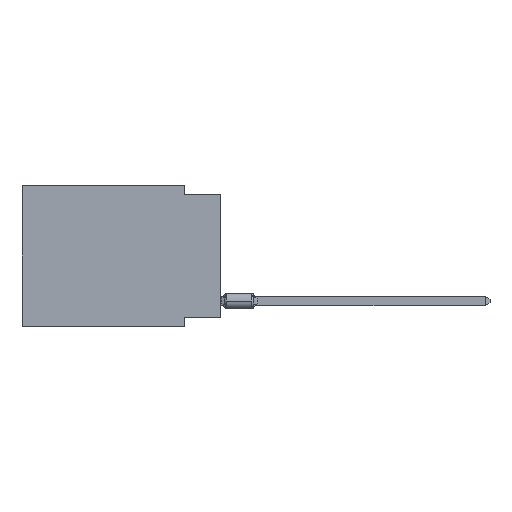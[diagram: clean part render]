
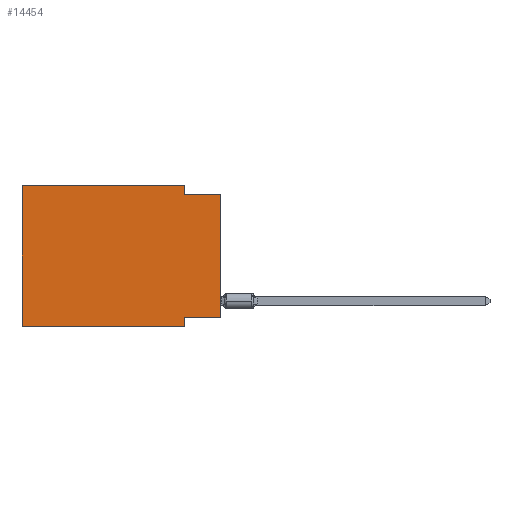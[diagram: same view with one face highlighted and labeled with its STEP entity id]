
A CAD part, left-side view. The second image highlights one B-rep face of the part: STEP entity #14454.
In plain terms, the highlighted planar face has unit normal (-1, 0, 0).
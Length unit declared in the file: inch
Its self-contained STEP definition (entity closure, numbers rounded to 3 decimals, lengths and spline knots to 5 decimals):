
#303 = EDGE_CURVE ( 'NONE', #1095, #17325, #11922, .T. ) ;
#632 = FACE_OUTER_BOUND ( 'NONE', #4413, .T. ) ;
#1095 = VERTEX_POINT ( 'NONE', #11320 ) ;
#1522 = LINE ( 'NONE', #7000, #1815 ) ;
#1712 = LINE ( 'NONE', #7549, #11616 ) ;
#1807 = ORIENTED_EDGE ( 'NONE', *, *, #2919, .F. ) ;
#1812 = VECTOR ( 'NONE', #8270, 39.37008 ) ;
#1815 = VECTOR ( 'NONE', #12707, 39.37008 ) ;
#2577 = VERTEX_POINT ( 'NONE', #18009 ) ;
#2919 = EDGE_CURVE ( 'NONE', #2577, #14890, #9937, .T. ) ;
#3273 = DIRECTION ( 'NONE',  ( 0., -1., 0. ) ) ;
#3311 = VERTEX_POINT ( 'NONE', #13706 ) ;
#3326 = DIRECTION ( 'NONE',  ( 0., 0., -1. ) ) ;
#3570 = EDGE_CURVE ( 'NONE', #8367, #17325, #12028, .T. ) ;
#3750 = CARTESIAN_POINT ( 'NONE',  ( 0., 0.55, 0. ) ) ;
#3968 = VECTOR ( 'NONE', #3326, 39.37008 ) ;
#4181 = CARTESIAN_POINT ( 'NONE',  ( 0., 0.55, 0. ) ) ;
#4274 = AXIS2_PLACEMENT_3D ( 'NONE', #6189, #11814, #7675 ) ;
#4413 = EDGE_LOOP ( 'NONE', ( #11760, #4896, #13779, #1807, #5230, #10850, #8039, #18053 ) ) ;
#4896 = ORIENTED_EDGE ( 'NONE', *, *, #3570, .F. ) ;
#5221 = LINE ( 'NONE', #3750, #11093 ) ;
#5230 = ORIENTED_EDGE ( 'NONE', *, *, #11577, .F. ) ;
#5623 = CARTESIAN_POINT ( 'NONE',  ( 0., 0.1, -0.025 ) ) ;
#6189 = CARTESIAN_POINT ( 'NONE',  ( 0., 0.55, 0. ) ) ;
#6210 = CARTESIAN_POINT ( 'NONE',  ( 0., 0., -0.025 ) ) ;
#6485 = CARTESIAN_POINT ( 'NONE',  ( 0., 0.1, -0.39 ) ) ;
#7000 = CARTESIAN_POINT ( 'NONE',  ( 0., 0., -0.365 ) ) ;
#7178 = EDGE_CURVE ( 'NONE', #14890, #8367, #8144, .T. ) ;
#7549 = CARTESIAN_POINT ( 'NONE',  ( 0., 0.55, -0.39 ) ) ;
#7631 = EDGE_CURVE ( 'NONE', #1095, #3311, #1522, .T. ) ;
#7675 = DIRECTION ( 'NONE',  ( 0., 0., -1. ) ) ;
#7762 = VECTOR ( 'NONE', #16100, 39.37008 ) ;
#8039 = ORIENTED_EDGE ( 'NONE', *, *, #10539, .F. ) ;
#8144 = LINE ( 'NONE', #12377, #14520 ) ;
#8172 = VERTEX_POINT ( 'NONE', #9076 ) ;
#8270 = DIRECTION ( 'NONE',  ( 0., -1., 0. ) ) ;
#8277 = CARTESIAN_POINT ( 'NONE',  ( 0., 0.1, 0. ) ) ;
#8367 = VERTEX_POINT ( 'NONE', #5623 ) ;
#9076 = CARTESIAN_POINT ( 'NONE',  ( 0., 0.55, -0.39 ) ) ;
#9250 = CARTESIAN_POINT ( 'NONE',  ( 0., 0., -0.025 ) ) ;
#9424 = DIRECTION ( 'NONE',  ( 0., 0., 1. ) ) ;
#9937 = LINE ( 'NONE', #4181, #1812 ) ;
#10187 = EDGE_CURVE ( 'NONE', #8172, #16349, #1712, .T. ) ;
#10346 = PLANE ( 'NONE',  #4274 ) ;
#10539 = EDGE_CURVE ( 'NONE', #3311, #16349, #13131, .T. ) ;
#10850 = ORIENTED_EDGE ( 'NONE', *, *, #10187, .T. ) ;
#10992 = DIRECTION ( 'NONE',  ( 0., 0., -1. ) ) ;
#11093 = VECTOR ( 'NONE', #16233, 39.37008 ) ;
#11320 = CARTESIAN_POINT ( 'NONE',  ( 0., 0., -0.365 ) ) ;
#11577 = EDGE_CURVE ( 'NONE', #8172, #2577, #5221, .T. ) ;
#11616 = VECTOR ( 'NONE', #3273, 39.37008 ) ;
#11760 = ORIENTED_EDGE ( 'NONE', *, *, #303, .T. ) ;
#11814 = DIRECTION ( 'NONE',  ( 1., 0., 0. ) ) ;
#11922 = LINE ( 'NONE', #16355, #14073 ) ;
#12028 = LINE ( 'NONE', #6210, #7762 ) ;
#12377 = CARTESIAN_POINT ( 'NONE',  ( 0., 0.1, 0. ) ) ;
#12707 = DIRECTION ( 'NONE',  ( 0., 1., 0. ) ) ;
#13131 = LINE ( 'NONE', #6485, #3968 ) ;
#13706 = CARTESIAN_POINT ( 'NONE',  ( 0., 0.1, -0.365 ) ) ;
#13779 = ORIENTED_EDGE ( 'NONE', *, *, #7178, .F. ) ;
#14073 = VECTOR ( 'NONE', #9424, 39.37008 ) ;
#14454 = ADVANCED_FACE ( 'NONE', ( #632 ), #10346, .F. ) ;
#14520 = VECTOR ( 'NONE', #10992, 39.37008 ) ;
#14890 = VERTEX_POINT ( 'NONE', #8277 ) ;
#16100 = DIRECTION ( 'NONE',  ( 0., -1., 0. ) ) ;
#16233 = DIRECTION ( 'NONE',  ( 0., 0., 1. ) ) ;
#16349 = VERTEX_POINT ( 'NONE', #17691 ) ;
#16355 = CARTESIAN_POINT ( 'NONE',  ( 0., 0., 0. ) ) ;
#17325 = VERTEX_POINT ( 'NONE', #9250 ) ;
#17691 = CARTESIAN_POINT ( 'NONE',  ( 0., 0.1, -0.39 ) ) ;
#18009 = CARTESIAN_POINT ( 'NONE',  ( 0., 0.55, 0. ) ) ;
#18053 = ORIENTED_EDGE ( 'NONE', *, *, #7631, .F. ) ;
